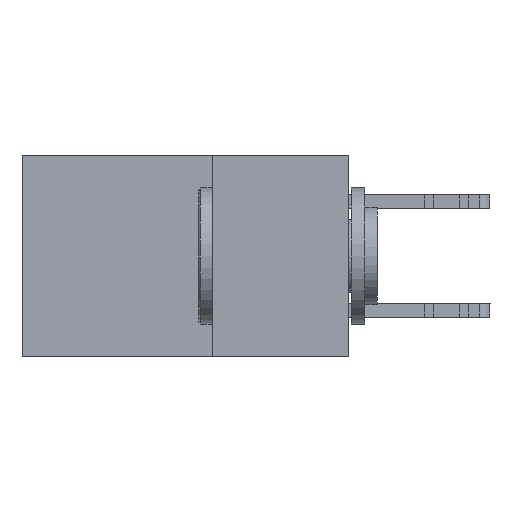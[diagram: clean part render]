
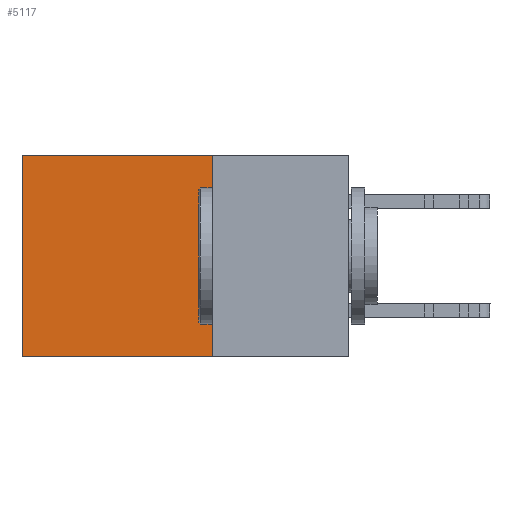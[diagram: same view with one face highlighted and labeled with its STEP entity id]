
A CAD part, left-side view. The second image highlights one B-rep face of the part: STEP entity #5117.
In plain terms, the highlighted planar face has unit normal (-1, 0, 0).
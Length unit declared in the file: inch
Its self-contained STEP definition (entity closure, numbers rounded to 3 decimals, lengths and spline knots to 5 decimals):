
#1649 = VECTOR ( 'NONE', #20684, 39.37008 ) ;
#1785 = EDGE_CURVE ( 'NONE', #26066, #24687, #7493, .T. ) ;
#4712 = EDGE_CURVE ( 'NONE', #16167, #24687, #13733, .T. ) ;
#5117 = ADVANCED_FACE ( 'NONE', ( #14362 ), #5726, .F. ) ;
#5726 = PLANE ( 'NONE',  #21973 ) ;
#6358 = VECTOR ( 'NONE', #10342, 39.37008 ) ;
#7420 = CARTESIAN_POINT ( 'NONE',  ( 0.2615, 0.25, -0.37 ) ) ;
#7493 = LINE ( 'NONE', #22733, #12297 ) ;
#7811 = DIRECTION ( 'NONE',  ( 0., 0., -1. ) ) ;
#7964 = EDGE_CURVE ( 'NONE', #14928, #26066, #18493, .T. ) ;
#8404 = CARTESIAN_POINT ( 'NONE',  ( 0.2615, 0.25, -0.37 ) ) ;
#10342 = DIRECTION ( 'NONE',  ( 0., 1., 0. ) ) ;
#10592 = CARTESIAN_POINT ( 'NONE',  ( 0.2615, 0.25, 0. ) ) ;
#10688 = DIRECTION ( 'NONE',  ( 0., 1., 0. ) ) ;
#10844 = EDGE_CURVE ( 'NONE', #14928, #16167, #18648, .T. ) ;
#12297 = VECTOR ( 'NONE', #23416, 39.37008 ) ;
#13244 = ORIENTED_EDGE ( 'NONE', *, *, #1785, .T. ) ;
#13733 = LINE ( 'NONE', #20533, #6358 ) ;
#14362 = FACE_OUTER_BOUND ( 'NONE', #26362, .T. ) ;
#14928 = VERTEX_POINT ( 'NONE', #20191 ) ;
#15324 = CARTESIAN_POINT ( 'NONE',  ( 0.2615, 0.6, 0. ) ) ;
#15950 = CARTESIAN_POINT ( 'NONE',  ( 0.2615, 0.25, -0.37 ) ) ;
#15998 = ORIENTED_EDGE ( 'NONE', *, *, #7964, .T. ) ;
#16167 = VERTEX_POINT ( 'NONE', #7420 ) ;
#16591 = ORIENTED_EDGE ( 'NONE', *, *, #4712, .F. ) ;
#17210 = VECTOR ( 'NONE', #10688, 39.37008 ) ;
#18493 = LINE ( 'NONE', #10592, #17210 ) ;
#18648 = LINE ( 'NONE', #8404, #1649 ) ;
#20077 = DIRECTION ( 'NONE',  ( 1., 0., 0. ) ) ;
#20191 = CARTESIAN_POINT ( 'NONE',  ( 0.2615, 0.25, 0. ) ) ;
#20533 = CARTESIAN_POINT ( 'NONE',  ( 0.2615, 0.25, -0.37 ) ) ;
#20684 = DIRECTION ( 'NONE',  ( 0., 0., -1. ) ) ;
#21973 = AXIS2_PLACEMENT_3D ( 'NONE', #15950, #20077, #7811 ) ;
#22733 = CARTESIAN_POINT ( 'NONE',  ( 0.2615, 0.6, -0.37 ) ) ;
#23416 = DIRECTION ( 'NONE',  ( 0., 0., -1. ) ) ;
#24668 = ORIENTED_EDGE ( 'NONE', *, *, #10844, .F. ) ;
#24687 = VERTEX_POINT ( 'NONE', #25222 ) ;
#25222 = CARTESIAN_POINT ( 'NONE',  ( 0.2615, 0.6, -0.37 ) ) ;
#26066 = VERTEX_POINT ( 'NONE', #15324 ) ;
#26362 = EDGE_LOOP ( 'NONE', ( #13244, #16591, #24668, #15998 ) ) ;
